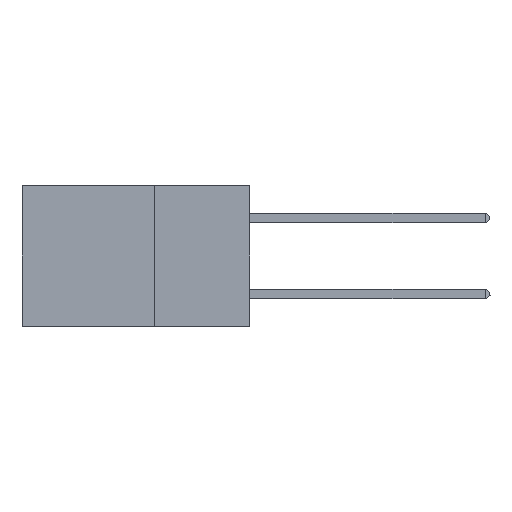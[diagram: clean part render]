
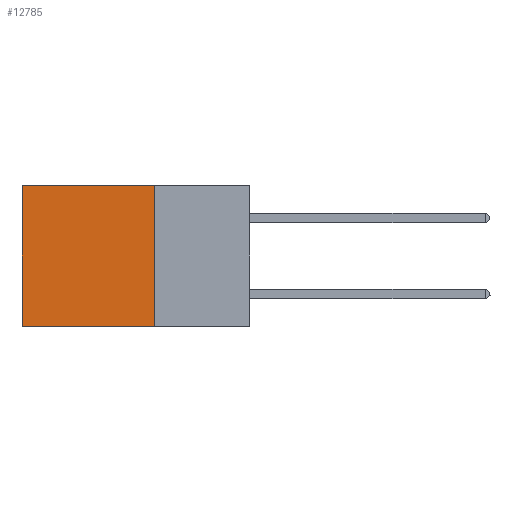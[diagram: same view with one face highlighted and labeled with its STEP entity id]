
A CAD part, left-side view. The second image highlights one B-rep face of the part: STEP entity #12785.
In plain terms, the highlighted planar face has unit normal (-1, 0, 0).
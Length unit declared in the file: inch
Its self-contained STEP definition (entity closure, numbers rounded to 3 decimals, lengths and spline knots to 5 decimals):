
#967 = CARTESIAN_POINT ( 'NONE',  ( 0.2875, 0.25, 0. ) ) ;
#968 = VERTEX_POINT ( 'NONE', #3658 ) ;
#1822 = DIRECTION ( 'NONE',  ( 1., 0., 0. ) ) ;
#2090 = CARTESIAN_POINT ( 'NONE',  ( 0.2875, 0.25, 0. ) ) ;
#2677 = EDGE_CURVE ( 'NONE', #5652, #968, #5670, .T. ) ;
#3472 = ORIENTED_EDGE ( 'NONE', *, *, #11137, .F. ) ;
#3592 = CARTESIAN_POINT ( 'NONE',  ( 0.2875, 0.6, 0. ) ) ;
#3658 = CARTESIAN_POINT ( 'NONE',  ( 0.2875, 0.6, 0. ) ) ;
#3782 = ORIENTED_EDGE ( 'NONE', *, *, #5953, .F. ) ;
#4088 = DIRECTION ( 'NONE',  ( 0., 1., 0. ) ) ;
#4165 = LINE ( 'NONE', #3592, #5805 ) ;
#4276 = EDGE_LOOP ( 'NONE', ( #7332, #3472, #3782, #6478 ) ) ;
#4395 = DIRECTION ( 'NONE',  ( 0., 0., -1. ) ) ;
#4511 = CARTESIAN_POINT ( 'NONE',  ( 0.2875, 0.25, 0. ) ) ;
#5373 = VERTEX_POINT ( 'NONE', #9902 ) ;
#5652 = VERTEX_POINT ( 'NONE', #2090 ) ;
#5670 = LINE ( 'NONE', #967, #15509 ) ;
#5805 = VECTOR ( 'NONE', #6161, 39.37008 ) ;
#5913 = EDGE_CURVE ( 'NONE', #968, #13793, #4165, .T. ) ;
#5953 = EDGE_CURVE ( 'NONE', #5652, #5373, #13627, .T. ) ;
#5992 = FACE_OUTER_BOUND ( 'NONE', #4276, .T. ) ;
#6161 = DIRECTION ( 'NONE',  ( 0., 0., -1. ) ) ;
#6386 = VECTOR ( 'NONE', #10108, 39.37008 ) ;
#6478 = ORIENTED_EDGE ( 'NONE', *, *, #2677, .T. ) ;
#6963 = AXIS2_PLACEMENT_3D ( 'NONE', #4511, #1822, #4395 ) ;
#7332 = ORIENTED_EDGE ( 'NONE', *, *, #5913, .T. ) ;
#9260 = VECTOR ( 'NONE', #12149, 39.37008 ) ;
#9390 = PLANE ( 'NONE',  #6963 ) ;
#9902 = CARTESIAN_POINT ( 'NONE',  ( 0.2875, 0.25, -0.37 ) ) ;
#10108 = DIRECTION ( 'NONE',  ( 0., 0., -1. ) ) ;
#10267 = LINE ( 'NONE', #14895, #9260 ) ;
#11137 = EDGE_CURVE ( 'NONE', #5373, #13793, #10267, .T. ) ;
#12149 = DIRECTION ( 'NONE',  ( 0., 1., 0. ) ) ;
#12572 = CARTESIAN_POINT ( 'NONE',  ( 0.2875, 0.25, 0. ) ) ;
#12785 = ADVANCED_FACE ( 'NONE', ( #5992 ), #9390, .F. ) ;
#13627 = LINE ( 'NONE', #12572, #6386 ) ;
#13793 = VERTEX_POINT ( 'NONE', #16496 ) ;
#14895 = CARTESIAN_POINT ( 'NONE',  ( 0.2875, 0.25, -0.37 ) ) ;
#15509 = VECTOR ( 'NONE', #4088, 39.37008 ) ;
#16496 = CARTESIAN_POINT ( 'NONE',  ( 0.2875, 0.6, -0.37 ) ) ;
